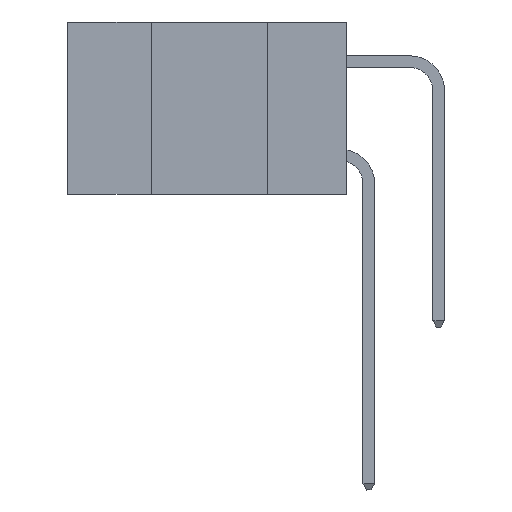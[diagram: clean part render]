
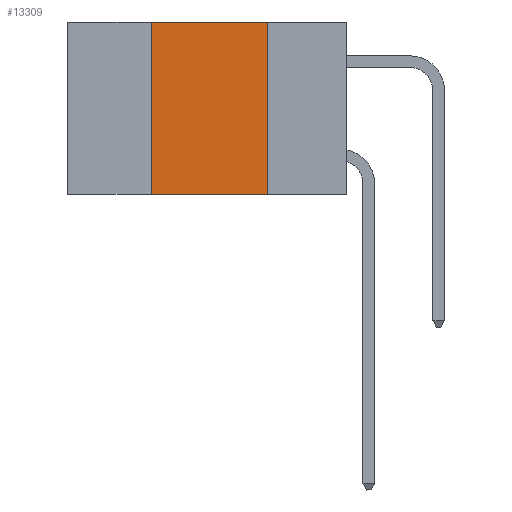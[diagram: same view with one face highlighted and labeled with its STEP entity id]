
A CAD part, left-side view. The second image highlights one B-rep face of the part: STEP entity #13309.
In plain terms, the highlighted planar face has unit normal (-1, 0, 0).
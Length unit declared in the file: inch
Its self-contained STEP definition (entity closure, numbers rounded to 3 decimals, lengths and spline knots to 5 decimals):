
#517 = EDGE_CURVE ( 'NONE', #7247, #5130, #1674, .T. ) ;
#612 = CARTESIAN_POINT ( 'NONE',  ( 0., 0.6, 0. ) ) ;
#721 = ORIENTED_EDGE ( 'NONE', *, *, #16339, .F. ) ;
#1674 = LINE ( 'NONE', #19474, #15513 ) ;
#1704 = VECTOR ( 'NONE', #7695, 39.37008 ) ;
#3008 = CARTESIAN_POINT ( 'NONE',  ( 0., 0.17, 0. ) ) ;
#3031 = ORIENTED_EDGE ( 'NONE', *, *, #14314, .F. ) ;
#3318 = EDGE_CURVE ( 'NONE', #14472, #12204, #13138, .T. ) ;
#4997 = CARTESIAN_POINT ( 'NONE',  ( 0., 0.42, 0. ) ) ;
#5031 = CARTESIAN_POINT ( 'NONE',  ( 0., 0.42, 0. ) ) ;
#5130 = VERTEX_POINT ( 'NONE', #12399 ) ;
#6045 = LINE ( 'NONE', #3008, #1704 ) ;
#6206 = LINE ( 'NONE', #5031, #16182 ) ;
#6769 = EDGE_LOOP ( 'NONE', ( #3031, #13647, #721, #9714 ) ) ;
#7071 = CARTESIAN_POINT ( 'NONE',  ( 0., 0.42, -0.37 ) ) ;
#7247 = VERTEX_POINT ( 'NONE', #4997 ) ;
#7695 = DIRECTION ( 'NONE',  ( 0., 0., -1. ) ) ;
#7870 = CARTESIAN_POINT ( 'NONE',  ( 0., 0.17, -0.37 ) ) ;
#8370 = DIRECTION ( 'NONE',  ( 1., 0., 0. ) ) ;
#8514 = FACE_OUTER_BOUND ( 'NONE', #6769, .T. ) ;
#9650 = PLANE ( 'NONE',  #10894 ) ;
#9712 = DIRECTION ( 'NONE',  ( 0., 0., 1. ) ) ;
#9714 = ORIENTED_EDGE ( 'NONE', *, *, #3318, .T. ) ;
#10894 = AXIS2_PLACEMENT_3D ( 'NONE', #612, #8370, #18991 ) ;
#12204 = VERTEX_POINT ( 'NONE', #7870 ) ;
#12399 = CARTESIAN_POINT ( 'NONE',  ( 0., 0.17, 0. ) ) ;
#13138 = LINE ( 'NONE', #13654, #18321 ) ;
#13309 = ADVANCED_FACE ( 'NONE', ( #8514 ), #9650, .F. ) ;
#13647 = ORIENTED_EDGE ( 'NONE', *, *, #517, .F. ) ;
#13654 = CARTESIAN_POINT ( 'NONE',  ( 0., 0.6, -0.37 ) ) ;
#14314 = EDGE_CURVE ( 'NONE', #5130, #12204, #6045, .T. ) ;
#14472 = VERTEX_POINT ( 'NONE', #7071 ) ;
#15513 = VECTOR ( 'NONE', #16584, 39.37008 ) ;
#16182 = VECTOR ( 'NONE', #9712, 39.37008 ) ;
#16339 = EDGE_CURVE ( 'NONE', #14472, #7247, #6206, .T. ) ;
#16584 = DIRECTION ( 'NONE',  ( 0., -1., 0. ) ) ;
#18321 = VECTOR ( 'NONE', #18328, 39.37008 ) ;
#18328 = DIRECTION ( 'NONE',  ( 0., -1., 0. ) ) ;
#18991 = DIRECTION ( 'NONE',  ( 0., 0., -1. ) ) ;
#19474 = CARTESIAN_POINT ( 'NONE',  ( 0., 0.6, 0. ) ) ;
